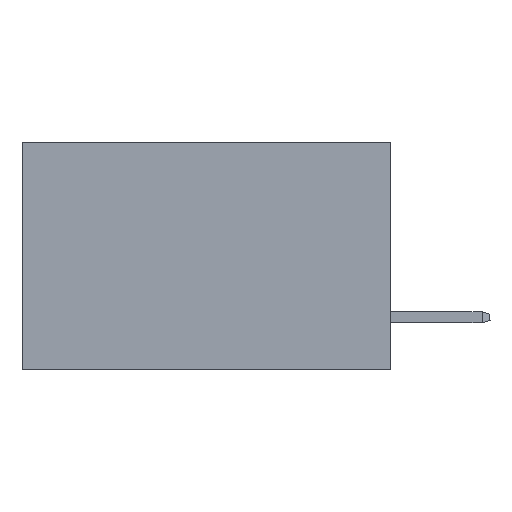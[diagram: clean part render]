
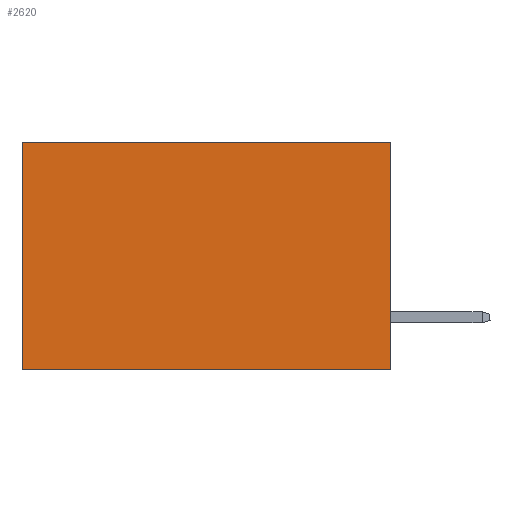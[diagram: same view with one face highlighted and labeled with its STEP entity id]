
A CAD part, left-side view. The second image highlights one B-rep face of the part: STEP entity #2620.
In plain terms, the highlighted planar face has unit normal (-1, 0, 0).
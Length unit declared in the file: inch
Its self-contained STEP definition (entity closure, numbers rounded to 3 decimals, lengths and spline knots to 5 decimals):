
#964 = DIRECTION ( 'NONE',  ( 0., 0., -1. ) ) ;
#984 = EDGE_CURVE ( 'NONE', #11571, #11930, #20988, .T. ) ;
#1128 = FACE_OUTER_BOUND ( 'NONE', #20046, .T. ) ;
#2283 = PLANE ( 'NONE',  #10540 ) ;
#2620 = ADVANCED_FACE ( 'NONE', ( #1128 ), #2283, .F. ) ;
#3522 = VECTOR ( 'NONE', #9897, 39.37008 ) ;
#3987 = ORIENTED_EDGE ( 'NONE', *, *, #10216, .T. ) ;
#5149 = EDGE_CURVE ( 'NONE', #6149, #11930, #9296, .T. ) ;
#6011 = DIRECTION ( 'NONE',  ( 0., 0., -1. ) ) ;
#6149 = VERTEX_POINT ( 'NONE', #21315 ) ;
#6244 = CARTESIAN_POINT ( 'NONE',  ( 0.2875, 0., 0. ) ) ;
#6497 = DIRECTION ( 'NONE',  ( 0., 0., -1. ) ) ;
#7897 = VERTEX_POINT ( 'NONE', #12204 ) ;
#7925 = ORIENTED_EDGE ( 'NONE', *, *, #15653, .F. ) ;
#8024 = ORIENTED_EDGE ( 'NONE', *, *, #984, .T. ) ;
#8219 = CARTESIAN_POINT ( 'NONE',  ( 0.2875, 0., -0.37 ) ) ;
#9296 = LINE ( 'NONE', #8219, #3522 ) ;
#9897 = DIRECTION ( 'NONE',  ( 0., 1., 0. ) ) ;
#10216 = EDGE_CURVE ( 'NONE', #7897, #11571, #22698, .T. ) ;
#10540 = AXIS2_PLACEMENT_3D ( 'NONE', #11366, #21843, #6011 ) ;
#10582 = VECTOR ( 'NONE', #964, 39.37008 ) ;
#11366 = CARTESIAN_POINT ( 'NONE',  ( 0.2875, 0., 0. ) ) ;
#11571 = VERTEX_POINT ( 'NONE', #12127 ) ;
#11631 = CARTESIAN_POINT ( 'NONE',  ( 0.2875, 0.6, 0. ) ) ;
#11930 = VERTEX_POINT ( 'NONE', #12059 ) ;
#12059 = CARTESIAN_POINT ( 'NONE',  ( 0.2875, 0.6, -0.37 ) ) ;
#12127 = CARTESIAN_POINT ( 'NONE',  ( 0.2875, 0.6, 0. ) ) ;
#12204 = CARTESIAN_POINT ( 'NONE',  ( 0.2875, 0., 0. ) ) ;
#13343 = VECTOR ( 'NONE', #6497, 39.37008 ) ;
#13894 = LINE ( 'NONE', #6244, #10582 ) ;
#13977 = ORIENTED_EDGE ( 'NONE', *, *, #5149, .F. ) ;
#15653 = EDGE_CURVE ( 'NONE', #7897, #6149, #13894, .T. ) ;
#15978 = DIRECTION ( 'NONE',  ( 0., 1., 0. ) ) ;
#18092 = VECTOR ( 'NONE', #15978, 39.37008 ) ;
#20046 = EDGE_LOOP ( 'NONE', ( #8024, #13977, #7925, #3987 ) ) ;
#20290 = CARTESIAN_POINT ( 'NONE',  ( 0.2875, 0., 0. ) ) ;
#20988 = LINE ( 'NONE', #11631, #13343 ) ;
#21315 = CARTESIAN_POINT ( 'NONE',  ( 0.2875, 0., -0.37 ) ) ;
#21843 = DIRECTION ( 'NONE',  ( 1., 0., 0. ) ) ;
#22698 = LINE ( 'NONE', #20290, #18092 ) ;
